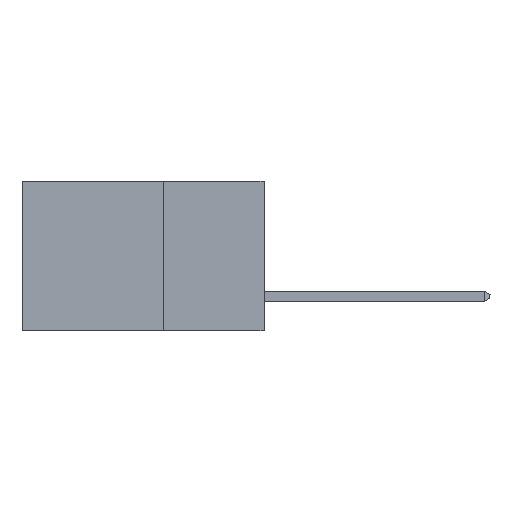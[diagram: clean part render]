
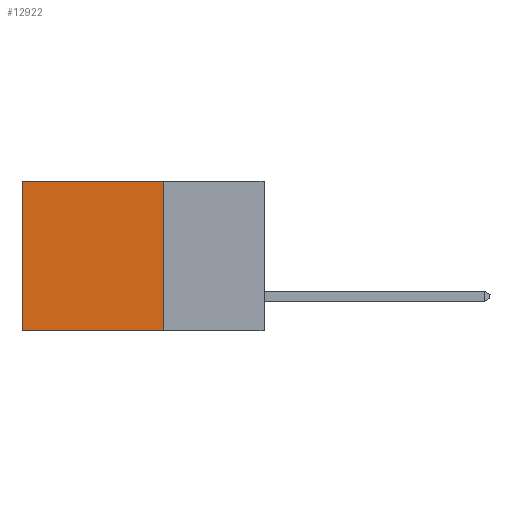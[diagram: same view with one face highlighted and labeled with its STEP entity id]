
A CAD part, left-side view. The second image highlights one B-rep face of the part: STEP entity #12922.
In plain terms, the highlighted planar face has unit normal (-1, 0, 0).
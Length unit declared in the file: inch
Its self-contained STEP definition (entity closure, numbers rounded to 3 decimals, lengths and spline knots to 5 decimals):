
#106 = DIRECTION ( 'NONE',  ( 0., 0., -1. ) ) ;
#233 = CARTESIAN_POINT ( 'NONE',  ( 0.298, 0.6, -0.37 ) ) ;
#287 = FACE_OUTER_BOUND ( 'NONE', #7547, .T. ) ;
#319 = EDGE_CURVE ( 'NONE', #9366, #15790, #5120, .T. ) ;
#1668 = VECTOR ( 'NONE', #9479, 39.37008 ) ;
#1748 = ORIENTED_EDGE ( 'NONE', *, *, #319, .T. ) ;
#3030 = CARTESIAN_POINT ( 'NONE',  ( 0.298, 0.25, -0.37 ) ) ;
#3167 = ORIENTED_EDGE ( 'NONE', *, *, #15061, .F. ) ;
#3968 = VERTEX_POINT ( 'NONE', #3030 ) ;
#4081 = DIRECTION ( 'NONE',  ( 0., 1., 0. ) ) ;
#5120 = LINE ( 'NONE', #15913, #1668 ) ;
#5263 = CARTESIAN_POINT ( 'NONE',  ( 0.298, 0.25, 0. ) ) ;
#6488 = PLANE ( 'NONE',  #8932 ) ;
#6590 = DIRECTION ( 'NONE',  ( 1., 0., 0. ) ) ;
#6612 = CARTESIAN_POINT ( 'NONE',  ( 0.298, 0.25, -0.37 ) ) ;
#6784 = CARTESIAN_POINT ( 'NONE',  ( 0.298, 0.25, 0. ) ) ;
#7026 = LINE ( 'NONE', #15634, #10129 ) ;
#7466 = ORIENTED_EDGE ( 'NONE', *, *, #11961, .F. ) ;
#7547 = EDGE_LOOP ( 'NONE', ( #10884, #3167, #7466, #1748 ) ) ;
#7845 = CARTESIAN_POINT ( 'NONE',  ( 0.298, 0.25, 0. ) ) ;
#8178 = VERTEX_POINT ( 'NONE', #233 ) ;
#8932 = AXIS2_PLACEMENT_3D ( 'NONE', #7845, #6590, #106 ) ;
#9366 = VERTEX_POINT ( 'NONE', #5263 ) ;
#9479 = DIRECTION ( 'NONE',  ( 0., 1., 0. ) ) ;
#10129 = VECTOR ( 'NONE', #13242, 39.37008 ) ;
#10197 = LINE ( 'NONE', #6784, #16207 ) ;
#10884 = ORIENTED_EDGE ( 'NONE', *, *, #13624, .T. ) ;
#11961 = EDGE_CURVE ( 'NONE', #9366, #3968, #10197, .T. ) ;
#12664 = LINE ( 'NONE', #6612, #13078 ) ;
#12922 = ADVANCED_FACE ( 'NONE', ( #287 ), #6488, .F. ) ;
#13078 = VECTOR ( 'NONE', #4081, 39.37008 ) ;
#13242 = DIRECTION ( 'NONE',  ( 0., 0., -1. ) ) ;
#13560 = DIRECTION ( 'NONE',  ( 0., 0., -1. ) ) ;
#13624 = EDGE_CURVE ( 'NONE', #15790, #8178, #7026, .T. ) ;
#15061 = EDGE_CURVE ( 'NONE', #3968, #8178, #12664, .T. ) ;
#15634 = CARTESIAN_POINT ( 'NONE',  ( 0.298, 0.6, 0. ) ) ;
#15790 = VERTEX_POINT ( 'NONE', #15885 ) ;
#15885 = CARTESIAN_POINT ( 'NONE',  ( 0.298, 0.6, 0. ) ) ;
#15913 = CARTESIAN_POINT ( 'NONE',  ( 0.298, 0.25, 0. ) ) ;
#16207 = VECTOR ( 'NONE', #13560, 39.37008 ) ;
